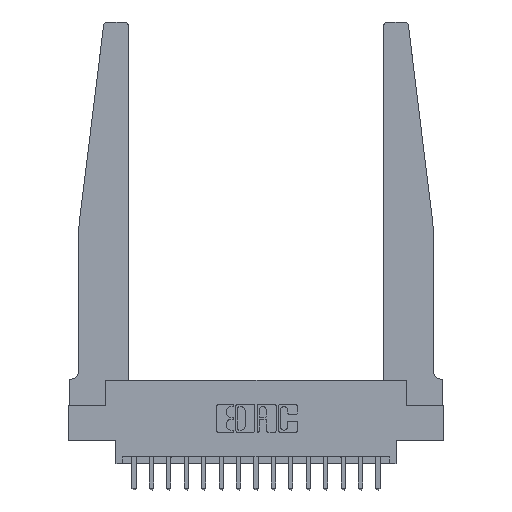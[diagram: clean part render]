
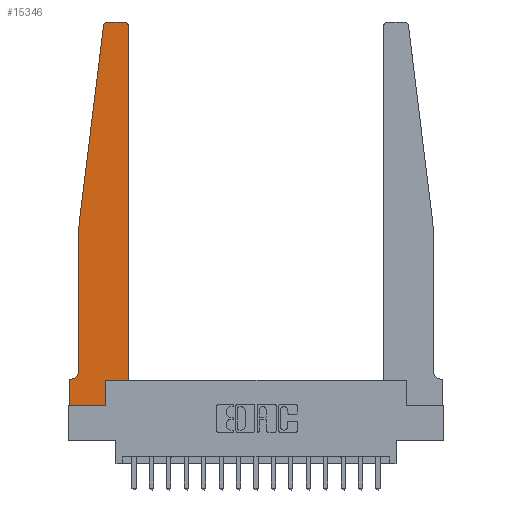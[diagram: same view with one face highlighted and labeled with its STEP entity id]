
A CAD part, top view. The second image highlights one B-rep face of the part: STEP entity #15346.
In plain terms, the highlighted planar face has unit normal (0, 0, 1).
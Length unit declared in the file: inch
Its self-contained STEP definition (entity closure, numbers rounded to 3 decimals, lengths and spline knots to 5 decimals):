
#69 = ORIENTED_EDGE ( 'NONE', *, *, #16857, .T. ) ;
#606 = VECTOR ( 'NONE', #9809, 39.37008 ) ;
#732 = LINE ( 'NONE', #12601, #9031 ) ;
#981 = VERTEX_POINT ( 'NONE', #5856 ) ;
#1041 = CARTESIAN_POINT ( 'NONE',  ( 0., 0., 0.37 ) ) ;
#1064 = LINE ( 'NONE', #18644, #1506 ) ;
#1096 = LINE ( 'NONE', #15900, #18612 ) ;
#1506 = VECTOR ( 'NONE', #8541, 39.37008 ) ;
#2093 = CARTESIAN_POINT ( 'NONE',  ( 0.24675, 2.72367, 0.37 ) ) ;
#2824 = LINE ( 'NONE', #18489, #7819 ) ;
#2908 = CARTESIAN_POINT ( 'NONE',  ( 0.2605, 0., 0.37 ) ) ;
#3072 = EDGE_CURVE ( 'NONE', #13268, #11372, #18134, .T. ) ;
#3741 = VERTEX_POINT ( 'NONE', #2908 ) ;
#3757 = CARTESIAN_POINT ( 'NONE',  ( 0.395, 2.72, 0.37 ) ) ;
#4503 = VERTEX_POINT ( 'NONE', #18874 ) ;
#4617 = CARTESIAN_POINT ( 'NONE',  ( 0., 0.1875, 0.37 ) ) ;
#4657 = EDGE_CURVE ( 'NONE', #9000, #3741, #17545, .T. ) ;
#4771 = ORIENTED_EDGE ( 'NONE', *, *, #15143, .T. ) ;
#4829 = CARTESIAN_POINT ( 'NONE',  ( 0.2605, 0.18, 0.37 ) ) ;
#5050 = DIRECTION ( 'NONE',  ( 0., -1., 0. ) ) ;
#5095 = AXIS2_PLACEMENT_3D ( 'NONE', #18439, #6906, #12525 ) ;
#5127 = EDGE_CURVE ( 'NONE', #3741, #8100, #13704, .T. ) ;
#5200 = DIRECTION ( 'NONE',  ( 0., 0., 1. ) ) ;
#5266 = LINE ( 'NONE', #1041, #11561 ) ;
#5597 = ORIENTED_EDGE ( 'NONE', *, *, #6283, .T. ) ;
#5724 = EDGE_CURVE ( 'NONE', #981, #6969, #16718, .T. ) ;
#5764 = VECTOR ( 'NONE', #5050, 39.37008 ) ;
#5783 = DIRECTION ( 'NONE',  ( 1., 0., 0. ) ) ;
#5856 = CARTESIAN_POINT ( 'NONE',  ( 0.27653, 2.75, 0.37 ) ) ;
#5908 = CIRCLE ( 'NONE', #12620, 0.05 ) ;
#6283 = EDGE_CURVE ( 'NONE', #11372, #4503, #5908, .T. ) ;
#6718 = VECTOR ( 'NONE', #12356, 39.37008 ) ;
#6906 = DIRECTION ( 'NONE',  ( 0., 0., 1. ) ) ;
#6969 = VERTEX_POINT ( 'NONE', #2093 ) ;
#7476 = DIRECTION ( 'NONE',  ( 1., 0., 0. ) ) ;
#7528 = DIRECTION ( 'NONE',  ( 1., 0., 0. ) ) ;
#7819 = VECTOR ( 'NONE', #11438, 39.37008 ) ;
#8058 = CARTESIAN_POINT ( 'NONE',  ( 0.015, 0.2375, 0.37 ) ) ;
#8100 = VERTEX_POINT ( 'NONE', #15671 ) ;
#8202 = ORIENTED_EDGE ( 'NONE', *, *, #13732, .T. ) ;
#8287 = CARTESIAN_POINT ( 'NONE',  ( 0.425, 0.18, 0.37 ) ) ;
#8365 = EDGE_CURVE ( 'NONE', #6969, #13268, #732, .T. ) ;
#8541 = DIRECTION ( 'NONE',  ( -1., 0., 0. ) ) ;
#8549 = DIRECTION ( 'NONE',  ( 1., 0., 0. ) ) ;
#8668 = CARTESIAN_POINT ( 'NONE',  ( 0., 0., 0.37 ) ) ;
#8910 = EDGE_CURVE ( 'NONE', #17373, #981, #2824, .T. ) ;
#9000 = VERTEX_POINT ( 'NONE', #8668 ) ;
#9031 = VECTOR ( 'NONE', #16706, 39.37008 ) ;
#9064 = CARTESIAN_POINT ( 'NONE',  ( 0., 0., 0.37 ) ) ;
#9114 = FACE_OUTER_BOUND ( 'NONE', #17629, .T. ) ;
#9247 = ORIENTED_EDGE ( 'NONE', *, *, #5724, .T. ) ;
#9351 = ORIENTED_EDGE ( 'NONE', *, *, #8910, .T. ) ;
#9504 = ORIENTED_EDGE ( 'NONE', *, *, #3072, .T. ) ;
#9751 = VERTEX_POINT ( 'NONE', #18515 ) ;
#9757 = DIRECTION ( 'NONE',  ( 0., -1., 0. ) ) ;
#9809 = DIRECTION ( 'NONE',  ( 0., 1., 0. ) ) ;
#10644 = ORIENTED_EDGE ( 'NONE', *, *, #8365, .T. ) ;
#11321 = VERTEX_POINT ( 'NONE', #17774 ) ;
#11372 = VERTEX_POINT ( 'NONE', #17967 ) ;
#11438 = DIRECTION ( 'NONE',  ( -1., 0., 0. ) ) ;
#11561 = VECTOR ( 'NONE', #9757, 39.37008 ) ;
#11869 = DIRECTION ( 'NONE',  ( 0., 0., 1. ) ) ;
#11920 = ORIENTED_EDGE ( 'NONE', *, *, #5127, .T. ) ;
#12212 = CIRCLE ( 'NONE', #13739, 0.03 ) ;
#12356 = DIRECTION ( 'NONE',  ( 0., 1., 0. ) ) ;
#12525 = DIRECTION ( 'NONE',  ( 1., 0., 0. ) ) ;
#12601 = CARTESIAN_POINT ( 'NONE',  ( 0.065, 1.25, 0.37 ) ) ;
#12620 = AXIS2_PLACEMENT_3D ( 'NONE', #8058, #17030, #15312 ) ;
#13268 = VERTEX_POINT ( 'NONE', #17728 ) ;
#13704 = LINE ( 'NONE', #4829, #6718 ) ;
#13732 = EDGE_CURVE ( 'NONE', #9751, #9000, #5266, .T. ) ;
#13739 = AXIS2_PLACEMENT_3D ( 'NONE', #3757, #5200, #8549 ) ;
#14029 = AXIS2_PLACEMENT_3D ( 'NONE', #4617, #11869, #7476 ) ;
#14206 = ORIENTED_EDGE ( 'NONE', *, *, #17646, .T. ) ;
#14291 = LINE ( 'NONE', #8287, #606 ) ;
#14509 = VERTEX_POINT ( 'NONE', #15267 ) ;
#14822 = PLANE ( 'NONE',  #14029 ) ;
#15108 = ORIENTED_EDGE ( 'NONE', *, *, #18214, .T. ) ;
#15143 = EDGE_CURVE ( 'NONE', #4503, #9751, #1064, .T. ) ;
#15267 = CARTESIAN_POINT ( 'NONE',  ( 0.425, 2.72, 0.37 ) ) ;
#15312 = DIRECTION ( 'NONE',  ( -1., 0., 0. ) ) ;
#15346 = ADVANCED_FACE ( 'NONE', ( #9114 ), #14822, .T. ) ;
#15350 = CARTESIAN_POINT ( 'NONE',  ( 0.065, 1.25, 0.37 ) ) ;
#15671 = CARTESIAN_POINT ( 'NONE',  ( 0.2605, 0.18, 0.37 ) ) ;
#15900 = CARTESIAN_POINT ( 'NONE',  ( 0.425, 0.18, 0.37 ) ) ;
#15941 = VECTOR ( 'NONE', #7528, 39.37008 ) ;
#16706 = DIRECTION ( 'NONE',  ( -0.122, -0.992, 0. ) ) ;
#16718 = CIRCLE ( 'NONE', #5095, 0.03 ) ;
#16857 = EDGE_CURVE ( 'NONE', #14509, #17373, #12212, .T. ) ;
#17030 = DIRECTION ( 'NONE',  ( 0., 0., -1. ) ) ;
#17373 = VERTEX_POINT ( 'NONE', #17834 ) ;
#17545 = LINE ( 'NONE', #9064, #15941 ) ;
#17629 = EDGE_LOOP ( 'NONE', ( #9351, #9247, #10644, #9504, #5597, #4771, #8202, #18147, #11920, #15108, #14206, #69 ) ) ;
#17646 = EDGE_CURVE ( 'NONE', #11321, #14509, #14291, .T. ) ;
#17728 = CARTESIAN_POINT ( 'NONE',  ( 0.065, 1.25, 0.37 ) ) ;
#17774 = CARTESIAN_POINT ( 'NONE',  ( 0.425, 0.18, 0.37 ) ) ;
#17834 = CARTESIAN_POINT ( 'NONE',  ( 0.395, 2.75, 0.37 ) ) ;
#17967 = CARTESIAN_POINT ( 'NONE',  ( 0.065, 0.2375, 0.37 ) ) ;
#18134 = LINE ( 'NONE', #15350, #5764 ) ;
#18147 = ORIENTED_EDGE ( 'NONE', *, *, #4657, .T. ) ;
#18214 = EDGE_CURVE ( 'NONE', #8100, #11321, #1096, .T. ) ;
#18439 = CARTESIAN_POINT ( 'NONE',  ( 0.27653, 2.72, 0.37 ) ) ;
#18489 = CARTESIAN_POINT ( 'NONE',  ( 0.25, 2.75, 0.37 ) ) ;
#18515 = CARTESIAN_POINT ( 'NONE',  ( 0., 0.1875, 0.37 ) ) ;
#18612 = VECTOR ( 'NONE', #5783, 39.37008 ) ;
#18644 = CARTESIAN_POINT ( 'NONE',  ( 0.065, 0.1875, 0.37 ) ) ;
#18874 = CARTESIAN_POINT ( 'NONE',  ( 0.015, 0.1875, 0.37 ) ) ;
